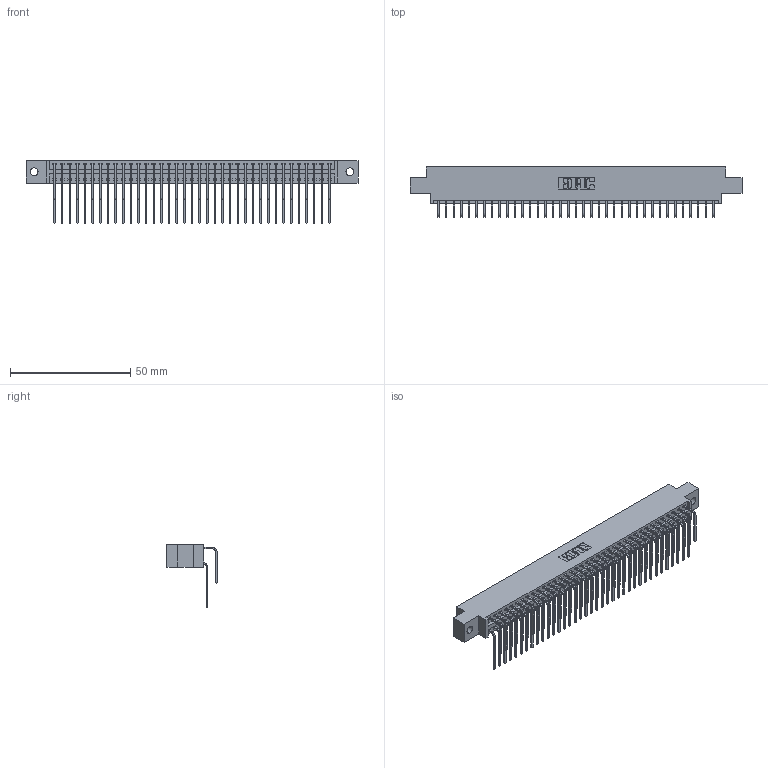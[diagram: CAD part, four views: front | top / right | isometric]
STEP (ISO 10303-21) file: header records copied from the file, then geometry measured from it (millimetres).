
FILE_DESCRIPTION (( 'STEP AP203' ), '1' );
FILE_NAME ('346-074-559-802.STEP', '2022-05-25T03:44:07', ( '' ), ( '' ), 'SwSTEP 2.0', 'SolidWorks 2020', '' );
FILE_SCHEMA (( 'CONFIG_CONTROL_DESIGN' ));
Length unit declared in the file: inch
Products named in the file (4): 345-292-001_558 559 Tail - 1; 346 Part_0.170 Offset - 0.128 Dia; 346-074-559-802; 345-292-001_559 Tail - 2
Assembly tree (75 placements, depth 2):
  346-074-559-802
    346 Part_0.170 Offset - 0.128 Dia
    345-292-001_558 559 Tail - 1  x37
    345-292-001_559 Tail - 2  x37
Bounding box: 138.05 x 20.89 x 26.16 mm (x, y, z)
Volume: 13658.2 mm3; surface area: 20653.9 mm2
Topology: 75 solids, 75 shells, 4122 faces, 12255 edges, 8070 vertices
Faces by surface type: plane 2818, cylinder 1304
Entity records: 26739 total; most frequent: CARTESIAN_POINT 4467, ORIENTED_EDGE 4350, DIRECTION 3959, EDGE_CURVE 2175, VECTOR 1855, LINE 1855, VERTEX_POINT 1446, AXIS2_PLACEMENT_3D 1052
